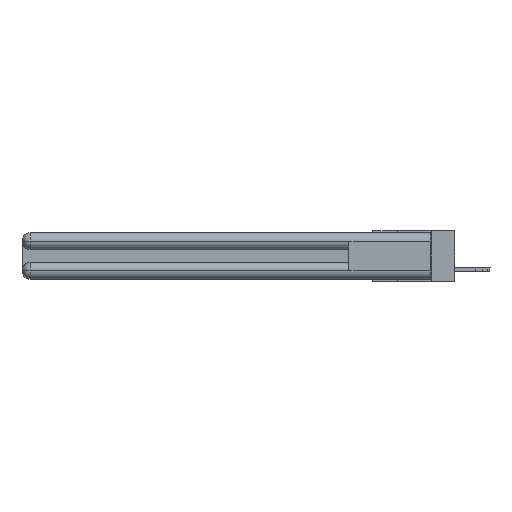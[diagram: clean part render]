
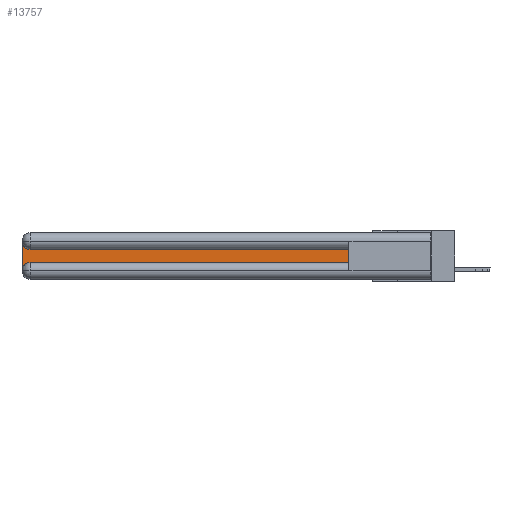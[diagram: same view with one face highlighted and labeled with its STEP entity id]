
A CAD part, left-side view. The second image highlights one B-rep face of the part: STEP entity #13757.
In plain terms, the highlighted planar face has unit normal (-1, 0, 0).
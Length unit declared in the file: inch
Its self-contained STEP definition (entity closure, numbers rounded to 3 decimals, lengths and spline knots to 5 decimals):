
#868 = VERTEX_POINT ( 'NONE', #16047 ) ;
#1583 = DIRECTION ( 'NONE',  ( 0., 0., 1. ) ) ;
#2270 = CARTESIAN_POINT ( 'NONE',  ( 0.075, 2.94, -0.2775 ) ) ;
#2683 = DIRECTION ( 'NONE',  ( 0., 0., -1. ) ) ;
#2896 = LINE ( 'NONE', #25184, #6076 ) ;
#3676 = ORIENTED_EDGE ( 'NONE', *, *, #24997, .T. ) ;
#4321 = DIRECTION ( 'NONE',  ( 0., 0., -1. ) ) ;
#4367 = VECTOR ( 'NONE', #20629, 39.37008 ) ;
#4593 = DIRECTION ( 'NONE',  ( 1., 0., 0. ) ) ;
#5101 = VERTEX_POINT ( 'NONE', #18475 ) ;
#5950 = ORIENTED_EDGE ( 'NONE', *, *, #24705, .T. ) ;
#6076 = VECTOR ( 'NONE', #2683, 39.37008 ) ;
#6293 = CARTESIAN_POINT ( 'NONE',  ( 0.075, 0.6, -0.1225 ) ) ;
#6308 = AXIS2_PLACEMENT_3D ( 'NONE', #18829, #4593, #6654 ) ;
#6440 = VERTEX_POINT ( 'NONE', #12610 ) ;
#6469 = EDGE_CURVE ( 'NONE', #5101, #16659, #11603, .T. ) ;
#6545 = ORIENTED_EDGE ( 'NONE', *, *, #6469, .T. ) ;
#6654 = DIRECTION ( 'NONE',  ( 0., 0., -1. ) ) ;
#6720 = LINE ( 'NONE', #17753, #21769 ) ;
#7182 = VERTEX_POINT ( 'NONE', #13411 ) ;
#11603 = CIRCLE ( 'NONE', #16706, 0.06 ) ;
#12610 = CARTESIAN_POINT ( 'NONE',  ( 0.075, 0.6, -0.2175 ) ) ;
#13350 = EDGE_CURVE ( 'NONE', #16659, #6440, #6720, .T. ) ;
#13411 = CARTESIAN_POINT ( 'NONE',  ( 0.075, 3., -0.0625 ) ) ;
#13425 = LINE ( 'NONE', #17847, #25086 ) ;
#13654 = AXIS2_PLACEMENT_3D ( 'NONE', #23274, #13863, #25916 ) ;
#13757 = ADVANCED_FACE ( 'NONE', ( #20821 ), #25445, .F. ) ;
#13863 = DIRECTION ( 'NONE',  ( 1., 0., 0. ) ) ;
#15541 = ORIENTED_EDGE ( 'NONE', *, *, #26193, .T. ) ;
#16047 = CARTESIAN_POINT ( 'NONE',  ( 0.075, 2.94, -0.1225 ) ) ;
#16547 = DIRECTION ( 'NONE',  ( 1., 0., 0. ) ) ;
#16659 = VERTEX_POINT ( 'NONE', #19203 ) ;
#16706 = AXIS2_PLACEMENT_3D ( 'NONE', #2270, #16547, #4321 ) ;
#17363 = EDGE_LOOP ( 'NONE', ( #21500, #3676, #15541, #6545, #21534, #5950 ) ) ;
#17688 = VERTEX_POINT ( 'NONE', #23206 ) ;
#17753 = CARTESIAN_POINT ( 'NONE',  ( 0.075, 0.6, -0.2175 ) ) ;
#17847 = CARTESIAN_POINT ( 'NONE',  ( 0.075, 0.6, -0.2175 ) ) ;
#18475 = CARTESIAN_POINT ( 'NONE',  ( 0.075, 3., -0.2775 ) ) ;
#18829 = CARTESIAN_POINT ( 'NONE',  ( 0.075, 2.94, -0.0625 ) ) ;
#19203 = CARTESIAN_POINT ( 'NONE',  ( 0.075, 2.94, -0.2175 ) ) ;
#19689 = LINE ( 'NONE', #6293, #4367 ) ;
#20629 = DIRECTION ( 'NONE',  ( 0., 1., 0. ) ) ;
#20821 = FACE_OUTER_BOUND ( 'NONE', #17363, .T. ) ;
#21500 = ORIENTED_EDGE ( 'NONE', *, *, #22444, .T. ) ;
#21534 = ORIENTED_EDGE ( 'NONE', *, *, #13350, .T. ) ;
#21738 = DIRECTION ( 'NONE',  ( 0., -1., 0. ) ) ;
#21769 = VECTOR ( 'NONE', #21738, 39.37008 ) ;
#22444 = EDGE_CURVE ( 'NONE', #17688, #868, #19689, .T. ) ;
#23206 = CARTESIAN_POINT ( 'NONE',  ( 0.075, 0.6, -0.1225 ) ) ;
#23274 = CARTESIAN_POINT ( 'NONE',  ( 0.075, 3., -0.1225 ) ) ;
#24705 = EDGE_CURVE ( 'NONE', #6440, #17688, #13425, .T. ) ;
#24744 = CIRCLE ( 'NONE', #6308, 0.06 ) ;
#24997 = EDGE_CURVE ( 'NONE', #868, #7182, #24744, .T. ) ;
#25086 = VECTOR ( 'NONE', #1583, 39.37008 ) ;
#25184 = CARTESIAN_POINT ( 'NONE',  ( 0.075, 3., -0.2175 ) ) ;
#25445 = PLANE ( 'NONE',  #13654 ) ;
#25916 = DIRECTION ( 'NONE',  ( 0., 0., -1. ) ) ;
#26193 = EDGE_CURVE ( 'NONE', #7182, #5101, #2896, .T. ) ;
